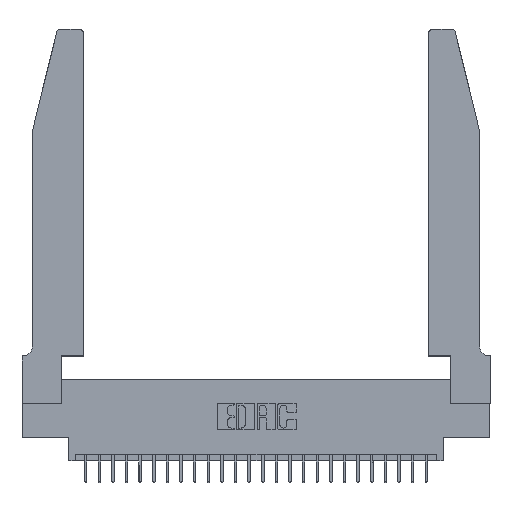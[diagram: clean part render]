
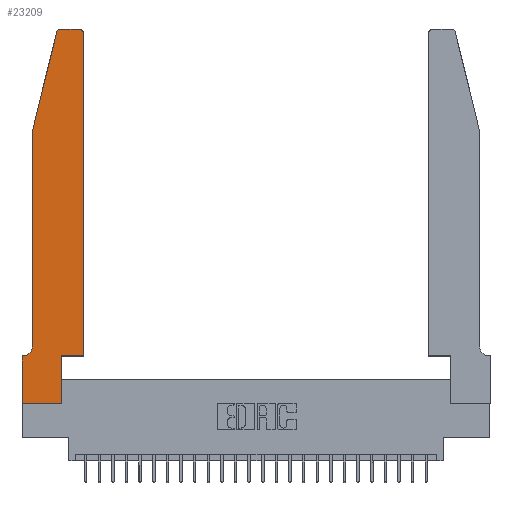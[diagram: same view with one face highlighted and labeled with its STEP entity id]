
A CAD part, top view. The second image highlights one B-rep face of the part: STEP entity #23209.
In plain terms, the highlighted planar face has unit normal (0, 0, 1).
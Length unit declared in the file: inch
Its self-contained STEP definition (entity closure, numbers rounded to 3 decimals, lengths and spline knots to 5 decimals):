
#398 = EDGE_CURVE ( 'NONE', #21813, #8279, #24677, .T. ) ;
#723 = AXIS2_PLACEMENT_3D ( 'NONE', #10517, #19238, #10780 ) ;
#895 = DIRECTION ( 'NONE',  ( 0., 1., 0. ) ) ;
#1177 = ORIENTED_EDGE ( 'NONE', *, *, #14064, .T. ) ;
#1237 = AXIS2_PLACEMENT_3D ( 'NONE', #5682, #10136, #10239 ) ;
#2035 = LINE ( 'NONE', #24380, #23931 ) ;
#2302 = CARTESIAN_POINT ( 'NONE',  ( 0.2865, 0.35, 0.37 ) ) ;
#2481 = CARTESIAN_POINT ( 'NONE',  ( 0.25487, 2.72718, 0.37 ) ) ;
#2982 = EDGE_CURVE ( 'NONE', #16717, #26869, #27059, .T. ) ;
#3146 = VERTEX_POINT ( 'NONE', #3179 ) ;
#3179 = CARTESIAN_POINT ( 'NONE',  ( 0.2865, 0., 0.37 ) ) ;
#3217 = VECTOR ( 'NONE', #11635, 39.37008 ) ;
#3364 = EDGE_CURVE ( 'NONE', #26869, #7393, #18120, .T. ) ;
#3377 = CARTESIAN_POINT ( 'NONE',  ( 0.0755, 0.35, 0.37 ) ) ;
#3421 = ORIENTED_EDGE ( 'NONE', *, *, #10252, .T. ) ;
#4062 = ORIENTED_EDGE ( 'NONE', *, *, #16047, .T. ) ;
#4093 = CARTESIAN_POINT ( 'NONE',  ( 0.4205, 2.72, 0.37 ) ) ;
#4174 = DIRECTION ( 'NONE',  ( 0., -1., 0. ) ) ;
#4194 = DIRECTION ( 'NONE',  ( 0., 1., 0. ) ) ;
#4454 = EDGE_CURVE ( 'NONE', #4799, #3146, #15091, .T. ) ;
#4799 = VERTEX_POINT ( 'NONE', #25014 ) ;
#5330 = DIRECTION ( 'NONE',  ( 0., -1., 0. ) ) ;
#5493 = CARTESIAN_POINT ( 'NONE',  ( 0.284, 2.72, 0.37 ) ) ;
#5682 = CARTESIAN_POINT ( 'NONE',  ( 0.0055, 0.42, 0.37 ) ) ;
#5844 = EDGE_CURVE ( 'NONE', #3146, #26480, #2035, .T. ) ;
#6015 = VERTEX_POINT ( 'NONE', #11936 ) ;
#6228 = DIRECTION ( 'NONE',  ( 0., 0., 1. ) ) ;
#6660 = CARTESIAN_POINT ( 'NONE',  ( 0.4505, 2.72, 0.37 ) ) ;
#6724 = CARTESIAN_POINT ( 'NONE',  ( 0.0755, 2., 0.37 ) ) ;
#6885 = CIRCLE ( 'NONE', #26262, 0.03 ) ;
#7002 = LINE ( 'NONE', #7404, #14324 ) ;
#7295 = LINE ( 'NONE', #23017, #25889 ) ;
#7393 = VERTEX_POINT ( 'NONE', #2481 ) ;
#7404 = CARTESIAN_POINT ( 'NONE',  ( 0.0755, 2., 0.37 ) ) ;
#7689 = AXIS2_PLACEMENT_3D ( 'NONE', #5493, #16543, #12435 ) ;
#8279 = VERTEX_POINT ( 'NONE', #6660 ) ;
#8553 = VECTOR ( 'NONE', #5330, 39.37008 ) ;
#8639 = ORIENTED_EDGE ( 'NONE', *, *, #398, .T. ) ;
#9185 = VECTOR ( 'NONE', #25618, 39.37008 ) ;
#9291 = CARTESIAN_POINT ( 'NONE',  ( 0.4205, 2.75, 0.37 ) ) ;
#9453 = VECTOR ( 'NONE', #19357, 39.37008 ) ;
#10136 = DIRECTION ( 'NONE',  ( 0., 0., -1. ) ) ;
#10239 = DIRECTION ( 'NONE',  ( -1., 0., 0. ) ) ;
#10252 = EDGE_CURVE ( 'NONE', #7393, #21595, #7002, .T. ) ;
#10517 = CARTESIAN_POINT ( 'NONE',  ( 0., 0.35, 0.37 ) ) ;
#10687 = CARTESIAN_POINT ( 'NONE',  ( 0.4505, 0.35, 0.37 ) ) ;
#10780 = DIRECTION ( 'NONE',  ( 1., 0., 0. ) ) ;
#11111 = ORIENTED_EDGE ( 'NONE', *, *, #4454, .T. ) ;
#11635 = DIRECTION ( 'NONE',  ( -1., 0., 0. ) ) ;
#11739 = VECTOR ( 'NONE', #4194, 39.37008 ) ;
#11936 = CARTESIAN_POINT ( 'NONE',  ( 0., 0.35, 0.37 ) ) ;
#12282 = CARTESIAN_POINT ( 'NONE',  ( 0.2605, 2.75, 0.37 ) ) ;
#12435 = DIRECTION ( 'NONE',  ( 1., 0., 0. ) ) ;
#12776 = CARTESIAN_POINT ( 'NONE',  ( 0.0755, 0.42, 0.37 ) ) ;
#13823 = DIRECTION ( 'NONE',  ( -0.239, -0.971, 0. ) ) ;
#14001 = ORIENTED_EDGE ( 'NONE', *, *, #20994, .T. ) ;
#14064 = EDGE_CURVE ( 'NONE', #22568, #23160, #15458, .T. ) ;
#14324 = VECTOR ( 'NONE', #13823, 39.37008 ) ;
#14873 = CARTESIAN_POINT ( 'NONE',  ( 0.0055, 0.35, 0.37 ) ) ;
#15091 = LINE ( 'NONE', #21438, #9453 ) ;
#15451 = VECTOR ( 'NONE', #18977, 39.37008 ) ;
#15458 = CIRCLE ( 'NONE', #1237, 0.07 ) ;
#16047 = EDGE_CURVE ( 'NONE', #23160, #6015, #18850, .T. ) ;
#16122 = EDGE_CURVE ( 'NONE', #21595, #22568, #24446, .T. ) ;
#16543 = DIRECTION ( 'NONE',  ( 0., 0., 1. ) ) ;
#16553 = EDGE_CURVE ( 'NONE', #26480, #21813, #24097, .T. ) ;
#16717 = VERTEX_POINT ( 'NONE', #9291 ) ;
#18105 = ORIENTED_EDGE ( 'NONE', *, *, #16122, .T. ) ;
#18120 = CIRCLE ( 'NONE', #7689, 0.03 ) ;
#18219 = ORIENTED_EDGE ( 'NONE', *, *, #16553, .T. ) ;
#18850 = LINE ( 'NONE', #3377, #3217 ) ;
#18863 = CARTESIAN_POINT ( 'NONE',  ( 0.4505, 0.35, 0.37 ) ) ;
#18977 = DIRECTION ( 'NONE',  ( -1., 0., 0. ) ) ;
#19125 = DIRECTION ( 'NONE',  ( 1., 0., 0. ) ) ;
#19238 = DIRECTION ( 'NONE',  ( 0., 0., 1. ) ) ;
#19357 = DIRECTION ( 'NONE',  ( 1., 0., 0. ) ) ;
#19682 = FACE_OUTER_BOUND ( 'NONE', #20804, .T. ) ;
#19826 = ORIENTED_EDGE ( 'NONE', *, *, #5844, .T. ) ;
#20795 = CARTESIAN_POINT ( 'NONE',  ( 0.284, 2.75, 0.37 ) ) ;
#20804 = EDGE_LOOP ( 'NONE', ( #25405, #27293, #3421, #18105, #1177, #4062, #14001, #11111, #19826, #18219, #8639, #26806 ) ) ;
#20994 = EDGE_CURVE ( 'NONE', #6015, #4799, #7295, .T. ) ;
#21218 = PLANE ( 'NONE',  #723 ) ;
#21438 = CARTESIAN_POINT ( 'NONE',  ( 0., 0., 0.37 ) ) ;
#21595 = VERTEX_POINT ( 'NONE', #6724 ) ;
#21813 = VERTEX_POINT ( 'NONE', #18863 ) ;
#22568 = VERTEX_POINT ( 'NONE', #12776 ) ;
#23017 = CARTESIAN_POINT ( 'NONE',  ( 0., 0., 0.37 ) ) ;
#23160 = VERTEX_POINT ( 'NONE', #14873 ) ;
#23209 = ADVANCED_FACE ( 'NONE', ( #19682 ), #21218, .T. ) ;
#23931 = VECTOR ( 'NONE', #895, 39.37008 ) ;
#24097 = LINE ( 'NONE', #10687, #9185 ) ;
#24380 = CARTESIAN_POINT ( 'NONE',  ( 0.2865, 0.35, 0.37 ) ) ;
#24446 = LINE ( 'NONE', #26469, #8553 ) ;
#24677 = LINE ( 'NONE', #25435, #11739 ) ;
#25014 = CARTESIAN_POINT ( 'NONE',  ( 0., 0., 0.37 ) ) ;
#25405 = ORIENTED_EDGE ( 'NONE', *, *, #2982, .T. ) ;
#25435 = CARTESIAN_POINT ( 'NONE',  ( 0.4505, 0.35, 0.37 ) ) ;
#25618 = DIRECTION ( 'NONE',  ( 1., 0., 0. ) ) ;
#25889 = VECTOR ( 'NONE', #4174, 39.37008 ) ;
#26262 = AXIS2_PLACEMENT_3D ( 'NONE', #4093, #6228, #19125 ) ;
#26318 = EDGE_CURVE ( 'NONE', #8279, #16717, #6885, .T. ) ;
#26469 = CARTESIAN_POINT ( 'NONE',  ( 0.0755, 2., 0.37 ) ) ;
#26480 = VERTEX_POINT ( 'NONE', #2302 ) ;
#26806 = ORIENTED_EDGE ( 'NONE', *, *, #26318, .T. ) ;
#26869 = VERTEX_POINT ( 'NONE', #20795 ) ;
#27059 = LINE ( 'NONE', #12282, #15451 ) ;
#27293 = ORIENTED_EDGE ( 'NONE', *, *, #3364, .T. ) ;
